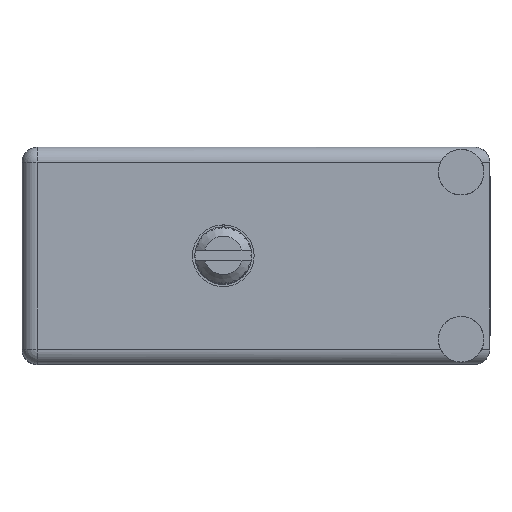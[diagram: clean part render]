
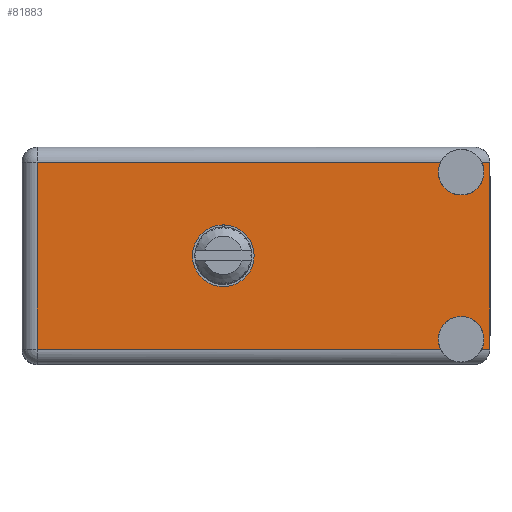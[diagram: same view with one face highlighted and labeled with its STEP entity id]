
A CAD part, top view. The second image highlights one B-rep face of the part: STEP entity #81883.
In plain terms, the highlighted face is planar.
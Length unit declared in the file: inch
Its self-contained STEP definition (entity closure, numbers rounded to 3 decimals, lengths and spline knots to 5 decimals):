
#6494 = EDGE_LOOP ( 'NONE', ( #61381, #59883 ) ) ;
#8599 = FACE_OUTER_BOUND ( 'NONE', #65484, .T. ) ;
#12859 = CIRCLE ( 'NONE', #156535, 0.075 ) ;
#14416 = CARTESIAN_POINT ( 'NONE',  ( -0.6125, 0.806, 0.3075 ) ) ;
#15510 = CARTESIAN_POINT ( 'NONE',  ( 0.85009, 0.806, -0.3075 ) ) ;
#17830 = DIRECTION ( 'NONE',  ( 0., 0., 1. ) ) ;
#18180 = VERTEX_POINT ( 'NONE', #14416 ) ;
#19794 = CIRCLE ( 'NONE', #134881, 0.1015 ) ;
#22513 = CARTESIAN_POINT ( 'NONE',  ( 0., 0.806, 0. ) ) ;
#23182 = DIRECTION ( 'NONE',  ( 0., 1., 0. ) ) ;
#23284 = CIRCLE ( 'NONE', #58804, 0.075 ) ;
#23538 = CARTESIAN_POINT ( 'NONE',  ( 0., 0.806, 0. ) ) ;
#25150 = PLANE ( 'NONE',  #157705 ) ;
#26746 = ORIENTED_EDGE ( 'NONE', *, *, #150070, .F. ) ;
#28544 = AXIS2_PLACEMENT_3D ( 'NONE', #155183, #108210, #156523 ) ;
#29390 = CARTESIAN_POINT ( 'NONE',  ( -0.6125, 0.806, -0.3575 ) ) ;
#33127 = CARTESIAN_POINT ( 'NONE',  ( 0.85009, 0.806, 0.3075 ) ) ;
#33892 = CARTESIAN_POINT ( 'NONE',  ( 0.8765, 0.806, -0.3075 ) ) ;
#34688 = DIRECTION ( 'NONE',  ( 0., 1., 0. ) ) ;
#34711 = CARTESIAN_POINT ( 'NONE',  ( -0.6125, 0.806, -0.3075 ) ) ;
#34845 = ORIENTED_EDGE ( 'NONE', *, *, #145351, .T. ) ;
#39969 = AXIS2_PLACEMENT_3D ( 'NONE', #93807, #34688, #17830 ) ;
#40256 = EDGE_CURVE ( 'NONE', #102212, #108834, #99272, .T. ) ;
#43466 = DIRECTION ( 'NONE',  ( 0., 0., 1. ) ) ;
#46165 = EDGE_CURVE ( 'NONE', #54091, #165070, #170463, .T. ) ;
#49350 = LINE ( 'NONE', #162431, #119290 ) ;
#54091 = VERTEX_POINT ( 'NONE', #33892 ) ;
#54174 = DIRECTION ( 'NONE',  ( -1., 0., 0. ) ) ;
#54621 = VECTOR ( 'NONE', #64067, 39.37008 ) ;
#55147 = CARTESIAN_POINT ( 'NONE',  ( 0.71491, 0.806, 0.3075 ) ) ;
#56233 = EDGE_CURVE ( 'NONE', #106438, #192680, #67373, .T. ) ;
#58771 = CARTESIAN_POINT ( 'NONE',  ( 0.7825, 0.806, -0.275 ) ) ;
#58804 = AXIS2_PLACEMENT_3D ( 'NONE', #58771, #166263, #136136 ) ;
#59883 = ORIENTED_EDGE ( 'NONE', *, *, #106419, .F. ) ;
#61381 = ORIENTED_EDGE ( 'NONE', *, *, #64637, .F. ) ;
#61545 = FACE_BOUND ( 'NONE', #6494, .T. ) ;
#61556 = CARTESIAN_POINT ( 'NONE',  ( 0.8765, 0.806, 0.3075 ) ) ;
#62073 = ORIENTED_EDGE ( 'NONE', *, *, #79969, .T. ) ;
#63216 = ORIENTED_EDGE ( 'NONE', *, *, #197104, .T. ) ;
#64067 = DIRECTION ( 'NONE',  ( 1., 0., 0. ) ) ;
#64637 = EDGE_CURVE ( 'NONE', #110713, #91355, #152816, .T. ) ;
#65484 = EDGE_LOOP ( 'NONE', ( #159852, #26746, #129643, #34845, #143917, #63216, #100903, #160174, #145015, #62073 ) ) ;
#67373 = LINE ( 'NONE', #133069, #103440 ) ;
#78431 = EDGE_CURVE ( 'NONE', #188042, #164622, #189718, .T. ) ;
#79969 = EDGE_CURVE ( 'NONE', #192680, #18180, #119867, .T. ) ;
#80323 = EDGE_CURVE ( 'NONE', #18180, #84859, #141168, .T. ) ;
#81883 = ADVANCED_FACE ( 'NONE', ( #61545, #8599 ), #25150, .T. ) ;
#84859 = VERTEX_POINT ( 'NONE', #55147 ) ;
#87691 = DIRECTION ( 'NONE',  ( 1., 0., 0. ) ) ;
#90312 = CARTESIAN_POINT ( 'NONE',  ( -0.6625, 0.806, -0.3075 ) ) ;
#91355 = VERTEX_POINT ( 'NONE', #156043 ) ;
#93807 = CARTESIAN_POINT ( 'NONE',  ( 0.7825, 0.806, 0.275 ) ) ;
#94525 = DIRECTION ( 'NONE',  ( 0., 1., 0. ) ) ;
#99272 = CIRCLE ( 'NONE', #28544, 0.075 ) ;
#100192 = CARTESIAN_POINT ( 'NONE',  ( 0.71491, 0.806, -0.3075 ) ) ;
#100482 = VECTOR ( 'NONE', #187913, 39.37008 ) ;
#100903 = ORIENTED_EDGE ( 'NONE', *, *, #40256, .F. ) ;
#101177 = CARTESIAN_POINT ( 'NONE',  ( -0.6625, 0.806, -0.3575 ) ) ;
#102212 = VERTEX_POINT ( 'NONE', #152348 ) ;
#103440 = VECTOR ( 'NONE', #141045, 39.37008 ) ;
#105101 = VECTOR ( 'NONE', #147759, 39.37008 ) ;
#105851 = AXIS2_PLACEMENT_3D ( 'NONE', #22513, #191935, #175787 ) ;
#106419 = EDGE_CURVE ( 'NONE', #91355, #110713, #19794, .T. ) ;
#106438 = VERTEX_POINT ( 'NONE', #100192 ) ;
#108210 = DIRECTION ( 'NONE',  ( 0., 1., 0. ) ) ;
#108834 = VERTEX_POINT ( 'NONE', #15510 ) ;
#110336 = VECTOR ( 'NONE', #43466, 39.37008 ) ;
#110713 = VERTEX_POINT ( 'NONE', #133708 ) ;
#116418 = DIRECTION ( 'NONE',  ( 0., 0., 1. ) ) ;
#119290 = VECTOR ( 'NONE', #87691, 39.37008 ) ;
#119867 = LINE ( 'NONE', #29390, #100482 ) ;
#121951 = LINE ( 'NONE', #90312, #105101 ) ;
#125587 = DIRECTION ( 'NONE',  ( 0., 0., 1. ) ) ;
#129643 = ORIENTED_EDGE ( 'NONE', *, *, #78431, .F. ) ;
#133069 = CARTESIAN_POINT ( 'NONE',  ( -0.6625, 0.806, -0.3075 ) ) ;
#133708 = CARTESIAN_POINT ( 'NONE',  ( 0., 0.806, 0.1015 ) ) ;
#134881 = AXIS2_PLACEMENT_3D ( 'NONE', #23538, #191606, #116418 ) ;
#136136 = DIRECTION ( 'NONE',  ( 0., 0., 1. ) ) ;
#138216 = CARTESIAN_POINT ( 'NONE',  ( 0.8765, 0.806, 0.3575 ) ) ;
#141045 = DIRECTION ( 'NONE',  ( -1., 0., 0. ) ) ;
#141168 = LINE ( 'NONE', #154791, #54621 ) ;
#142620 = EDGE_CURVE ( 'NONE', #106438, #102212, #23284, .T. ) ;
#143917 = ORIENTED_EDGE ( 'NONE', *, *, #46165, .F. ) ;
#145015 = ORIENTED_EDGE ( 'NONE', *, *, #56233, .T. ) ;
#145351 = EDGE_CURVE ( 'NONE', #188042, #165070, #49350, .T. ) ;
#147759 = DIRECTION ( 'NONE',  ( -1., 0., 0. ) ) ;
#150070 = EDGE_CURVE ( 'NONE', #164622, #84859, #12859, .T. ) ;
#152348 = CARTESIAN_POINT ( 'NONE',  ( 0.7825, 0.806, -0.2 ) ) ;
#152816 = CIRCLE ( 'NONE', #105851, 0.1015 ) ;
#154791 = CARTESIAN_POINT ( 'NONE',  ( 0.8765, 0.806, 0.3075 ) ) ;
#155183 = CARTESIAN_POINT ( 'NONE',  ( 0.7825, 0.806, -0.275 ) ) ;
#156043 = CARTESIAN_POINT ( 'NONE',  ( 0., 0.806, -0.1015 ) ) ;
#156523 = DIRECTION ( 'NONE',  ( 0., 0., 1. ) ) ;
#156535 = AXIS2_PLACEMENT_3D ( 'NONE', #186670, #94525, #125587 ) ;
#157705 = AXIS2_PLACEMENT_3D ( 'NONE', #101177, #23182, #54174 ) ;
#159852 = ORIENTED_EDGE ( 'NONE', *, *, #80323, .T. ) ;
#160174 = ORIENTED_EDGE ( 'NONE', *, *, #142620, .F. ) ;
#162431 = CARTESIAN_POINT ( 'NONE',  ( 0.8765, 0.806, 0.3075 ) ) ;
#164622 = VERTEX_POINT ( 'NONE', #190835 ) ;
#165070 = VERTEX_POINT ( 'NONE', #61556 ) ;
#166263 = DIRECTION ( 'NONE',  ( 0., 1., 0. ) ) ;
#170463 = LINE ( 'NONE', #138216, #110336 ) ;
#175787 = DIRECTION ( 'NONE',  ( 0., 0., 1. ) ) ;
#186670 = CARTESIAN_POINT ( 'NONE',  ( 0.7825, 0.806, 0.275 ) ) ;
#187913 = DIRECTION ( 'NONE',  ( 0., 0., 1. ) ) ;
#188042 = VERTEX_POINT ( 'NONE', #33127 ) ;
#189718 = CIRCLE ( 'NONE', #39969, 0.075 ) ;
#190835 = CARTESIAN_POINT ( 'NONE',  ( 0.7825, 0.806, 0.2 ) ) ;
#191606 = DIRECTION ( 'NONE',  ( 0., 1., 0. ) ) ;
#191935 = DIRECTION ( 'NONE',  ( 0., 1., 0. ) ) ;
#192680 = VERTEX_POINT ( 'NONE', #34711 ) ;
#197104 = EDGE_CURVE ( 'NONE', #54091, #108834, #121951, .T. ) ;
